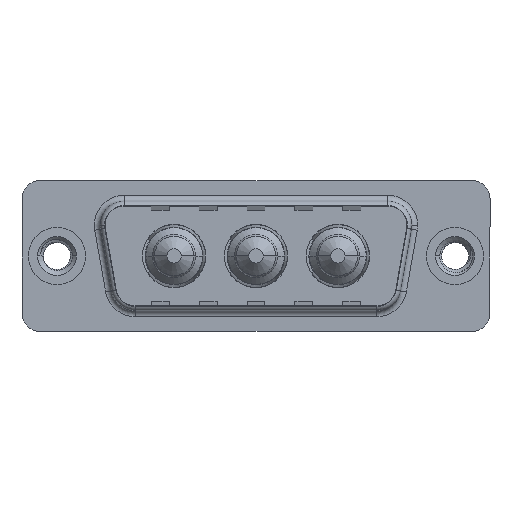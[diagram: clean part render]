
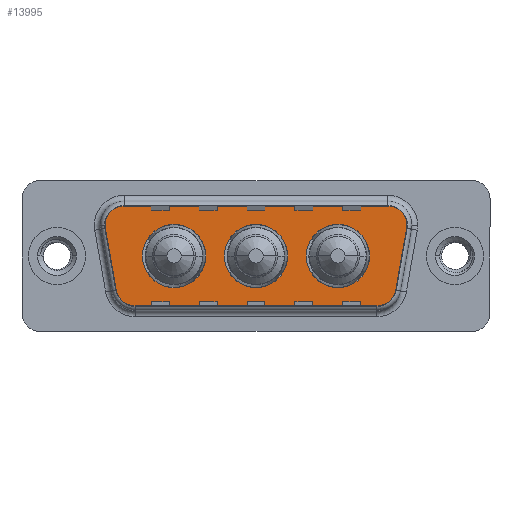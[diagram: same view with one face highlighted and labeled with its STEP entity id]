
A CAD part, top view. The second image highlights one B-rep face of the part: STEP entity #13995.
In plain terms, the highlighted planar face has unit normal (0, 0, 1).
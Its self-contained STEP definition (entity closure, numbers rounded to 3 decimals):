
#9 = CARTESIAN_POINT ( 'NONE',  ( 16.65, 0., 0. ) ) ;
#160 = ORIENTED_EDGE ( 'NONE', *, *, #9346, .F. ) ;
#210 = CARTESIAN_POINT ( 'NONE',  ( 5.411, 4.9, 0. ) ) ;
#265 = DIRECTION ( 'NONE',  ( -1., 0., 0. ) ) ;
#535 = VECTOR ( 'NONE', #265, 1000. ) ;
#558 = CARTESIAN_POINT ( 'NONE',  ( 6.434, -4.9, 0. ) ) ;
#562 = ORIENTED_EDGE ( 'NONE', *, *, #14054, .F. ) ;
#684 = CARTESIAN_POINT ( 'NONE',  ( 26.866, -4.9, 0. ) ) ;
#723 = DIRECTION ( 'NONE',  ( 0., 0., 1. ) ) ;
#787 = CIRCLE ( 'NONE', #1779, 2. ) ;
#826 = DIRECTION ( 'NONE',  ( 0.174, 0.985, 0. ) ) ;
#1057 = AXIS2_PLACEMENT_3D ( 'NONE', #14689, #14650, #14646 ) ;
#1216 = VECTOR ( 'NONE', #826, 1000. ) ;
#1228 = CIRCLE ( 'NONE', #1946, 2. ) ;
#1243 = ORIENTED_EDGE ( 'NONE', *, *, #7879, .F. ) ;
#1320 = CARTESIAN_POINT ( 'NONE',  ( 27.889, 4.9, 0. ) ) ;
#1779 = AXIS2_PLACEMENT_3D ( 'NONE', #15324, #15310, #15288 ) ;
#1879 = DIRECTION ( 'NONE',  ( 1., 0., 0. ) ) ;
#1946 = AXIS2_PLACEMENT_3D ( 'NONE', #11433, #4118, #12653 ) ;
#2027 = CARTESIAN_POINT ( 'NONE',  ( 29.859, 2.553, 0. ) ) ;
#2091 = DIRECTION ( 'NONE',  ( 0., 0., 1. ) ) ;
#2092 = ORIENTED_EDGE ( 'NONE', *, *, #9928, .T. ) ;
#2389 = CARTESIAN_POINT ( 'NONE',  ( 5.411, 2.9, 0. ) ) ;
#2414 = ORIENTED_EDGE ( 'NONE', *, *, #2459, .F. ) ;
#2451 = CIRCLE ( 'NONE', #11569, 2.65 ) ;
#2459 = EDGE_CURVE ( 'NONE', #6737, #3568, #2959, .T. ) ;
#2543 = AXIS2_PLACEMENT_3D ( 'NONE', #2389, #6578, #6451 ) ;
#2721 = CARTESIAN_POINT ( 'NONE',  ( 26.15, 0., 0. ) ) ;
#2831 = DIRECTION ( 'NONE',  ( 0., 0., 1. ) ) ;
#2881 = AXIS2_PLACEMENT_3D ( 'NONE', #9, #5529, #13984 ) ;
#2959 = CIRCLE ( 'NONE', #15672, 2.65 ) ;
#3270 = VERTEX_POINT ( 'NONE', #15400 ) ;
#3435 = LINE ( 'NONE', #210, #535 ) ;
#3568 = VERTEX_POINT ( 'NONE', #5178 ) ;
#3673 = VERTEX_POINT ( 'NONE', #5224 ) ;
#3824 = CIRCLE ( 'NONE', #2881, 2.65 ) ;
#3828 = EDGE_LOOP ( 'NONE', ( #7316, #160 ) ) ;
#4067 = CARTESIAN_POINT ( 'NONE',  ( 3.441, 2.553, 0. ) ) ;
#4118 = DIRECTION ( 'NONE',  ( 0., 0., 1. ) ) ;
#4193 = ORIENTED_EDGE ( 'NONE', *, *, #6285, .T. ) ;
#4564 = FACE_BOUND ( 'NONE', #13454, .T. ) ;
#4695 = ORIENTED_EDGE ( 'NONE', *, *, #15006, .T. ) ;
#4740 = DIRECTION ( 'NONE',  ( 0., 0., 1. ) ) ;
#4900 = LINE ( 'NONE', #2027, #1216 ) ;
#5067 = CARTESIAN_POINT ( 'NONE',  ( 4.464, -3.247, 0. ) ) ;
#5170 = LINE ( 'NONE', #11577, #14444 ) ;
#5178 = CARTESIAN_POINT ( 'NONE',  ( 7.15, 0., 0. ) ) ;
#5224 = CARTESIAN_POINT ( 'NONE',  ( 14., 0., 0. ) ) ;
#5529 = DIRECTION ( 'NONE',  ( 0., 0., 1. ) ) ;
#5687 = CARTESIAN_POINT ( 'NONE',  ( 9.8, 0., 0. ) ) ;
#6285 = EDGE_CURVE ( 'NONE', #8178, #7769, #6385, .T. ) ;
#6385 = CIRCLE ( 'NONE', #2543, 2. ) ;
#6451 = DIRECTION ( 'NONE',  ( 1., 0., 0. ) ) ;
#6578 = DIRECTION ( 'NONE',  ( 0., 0., 1. ) ) ;
#6622 = CARTESIAN_POINT ( 'NONE',  ( 20.85, 0., 0. ) ) ;
#6737 = VERTEX_POINT ( 'NONE', #14676 ) ;
#6766 = CARTESIAN_POINT ( 'NONE',  ( 9.8, 0., 0. ) ) ;
#7316 = ORIENTED_EDGE ( 'NONE', *, *, #11555, .F. ) ;
#7460 = EDGE_CURVE ( 'NONE', #11026, #12460, #11541, .T. ) ;
#7506 = EDGE_LOOP ( 'NONE', ( #2414, #562 ) ) ;
#7604 = CARTESIAN_POINT ( 'NONE',  ( 5.411, 4.9, 0. ) ) ;
#7656 = ORIENTED_EDGE ( 'NONE', *, *, #11028, .T. ) ;
#7769 = VERTEX_POINT ( 'NONE', #4067 ) ;
#7793 = EDGE_CURVE ( 'NONE', #10561, #12694, #787, .T. ) ;
#7811 = FACE_BOUND ( 'NONE', #7506, .T. ) ;
#7879 = EDGE_CURVE ( 'NONE', #3673, #3270, #12298, .T. ) ;
#8046 = DIRECTION ( 'NONE',  ( 1., 0., 0. ) ) ;
#8098 = CARTESIAN_POINT ( 'NONE',  ( 23.5, 0., 0. ) ) ;
#8178 = VERTEX_POINT ( 'NONE', #7604 ) ;
#8218 = FACE_OUTER_BOUND ( 'NONE', #14787, .T. ) ;
#8435 = VERTEX_POINT ( 'NONE', #2721 ) ;
#8458 = ORIENTED_EDGE ( 'NONE', *, *, #14545, .T. ) ;
#8600 = FACE_BOUND ( 'NONE', #3828, .T. ) ;
#8952 = PLANE ( 'NONE',  #14253 ) ;
#9040 = VERTEX_POINT ( 'NONE', #6622 ) ;
#9142 = CIRCLE ( 'NONE', #9356, 2. ) ;
#9193 = VERTEX_POINT ( 'NONE', #1320 ) ;
#9204 = AXIS2_PLACEMENT_3D ( 'NONE', #13824, #13725, #13697 ) ;
#9298 = DIRECTION ( 'NONE',  ( 1., 0., 0. ) ) ;
#9346 = EDGE_CURVE ( 'NONE', #9040, #8435, #11849, .T. ) ;
#9356 = AXIS2_PLACEMENT_3D ( 'NONE', #12038, #4740, #13241 ) ;
#9700 = VERTEX_POINT ( 'NONE', #13318 ) ;
#9919 = VECTOR ( 'NONE', #1879, 1000. ) ;
#9928 = EDGE_CURVE ( 'NONE', #7769, #10561, #5170, .T. ) ;
#9955 = VERTEX_POINT ( 'NONE', #11486 ) ;
#10129 = CARTESIAN_POINT ( 'NONE',  ( 26.866, -2.9, 0. ) ) ;
#10206 = ORIENTED_EDGE ( 'NONE', *, *, #7793, .T. ) ;
#10482 = CARTESIAN_POINT ( 'NONE',  ( 28.836, -3.247, 0. ) ) ;
#10561 = VERTEX_POINT ( 'NONE', #5067 ) ;
#10887 = ORIENTED_EDGE ( 'NONE', *, *, #14657, .T. ) ;
#11026 = VERTEX_POINT ( 'NONE', #684 ) ;
#11028 = EDGE_CURVE ( 'NONE', #12694, #11026, #13148, .T. ) ;
#11049 = EDGE_CURVE ( 'NONE', #9193, #8178, #3435, .T. ) ;
#11053 = ORIENTED_EDGE ( 'NONE', *, *, #11049, .T. ) ;
#11063 = EDGE_CURVE ( 'NONE', #3270, #3673, #3824, .T. ) ;
#11163 = ORIENTED_EDGE ( 'NONE', *, *, #11063, .F. ) ;
#11433 = CARTESIAN_POINT ( 'NONE',  ( 27.889, 2.9, 0. ) ) ;
#11446 = CIRCLE ( 'NONE', #15084, 2.65 ) ;
#11486 = CARTESIAN_POINT ( 'NONE',  ( 29.889, 2.9, 0. ) ) ;
#11539 = DIRECTION ( 'NONE',  ( 0.174, -0.985, 0. ) ) ;
#11541 = CIRCLE ( 'NONE', #13609, 2. ) ;
#11555 = EDGE_CURVE ( 'NONE', #8435, #9040, #2451, .T. ) ;
#11569 = AXIS2_PLACEMENT_3D ( 'NONE', #8098, #723, #9298 ) ;
#11577 = CARTESIAN_POINT ( 'NONE',  ( 3.441, 2.553, 0. ) ) ;
#11587 = DIRECTION ( 'NONE',  ( 1., 0., 0. ) ) ;
#11849 = CIRCLE ( 'NONE', #1057, 2.65 ) ;
#12038 = CARTESIAN_POINT ( 'NONE',  ( 27.889, 2.9, 0. ) ) ;
#12228 = ORIENTED_EDGE ( 'NONE', *, *, #7460, .T. ) ;
#12298 = CIRCLE ( 'NONE', #9204, 2.65 ) ;
#12460 = VERTEX_POINT ( 'NONE', #10482 ) ;
#12653 = DIRECTION ( 'NONE',  ( -1., 0., 0. ) ) ;
#12694 = VERTEX_POINT ( 'NONE', #14528 ) ;
#13148 = LINE ( 'NONE', #558, #9919 ) ;
#13241 = DIRECTION ( 'NONE',  ( -1., 0., 0. ) ) ;
#13318 = CARTESIAN_POINT ( 'NONE',  ( 29.859, 2.553, 0. ) ) ;
#13454 = EDGE_LOOP ( 'NONE', ( #11163, #1243 ) ) ;
#13609 = AXIS2_PLACEMENT_3D ( 'NONE', #14417, #14235, #14141 ) ;
#13697 = DIRECTION ( 'NONE',  ( 1., 0., 0. ) ) ;
#13725 = DIRECTION ( 'NONE',  ( 0., 0., 1. ) ) ;
#13824 = CARTESIAN_POINT ( 'NONE',  ( 16.65, 0., 0. ) ) ;
#13984 = DIRECTION ( 'NONE',  ( 1., 0., 0. ) ) ;
#13995 = ADVANCED_FACE ( 'NONE', ( #4564, #8600, #7811, #8218 ), #8952, .T. ) ;
#14054 = EDGE_CURVE ( 'NONE', #3568, #6737, #11446, .T. ) ;
#14141 = DIRECTION ( 'NONE',  ( 1., 0., 0. ) ) ;
#14235 = DIRECTION ( 'NONE',  ( 0., 0., 1. ) ) ;
#14253 = AXIS2_PLACEMENT_3D ( 'NONE', #10129, #2831, #11587 ) ;
#14417 = CARTESIAN_POINT ( 'NONE',  ( 26.866, -2.9, 0. ) ) ;
#14444 = VECTOR ( 'NONE', #11539, 1000. ) ;
#14528 = CARTESIAN_POINT ( 'NONE',  ( 6.434, -4.9, 0. ) ) ;
#14545 = EDGE_CURVE ( 'NONE', #9700, #9955, #1228, .T. ) ;
#14646 = DIRECTION ( 'NONE',  ( 1., 0., 0. ) ) ;
#14650 = DIRECTION ( 'NONE',  ( 0., 0., 1. ) ) ;
#14657 = EDGE_CURVE ( 'NONE', #9955, #9193, #9142, .T. ) ;
#14676 = CARTESIAN_POINT ( 'NONE',  ( 12.45, 0., 0. ) ) ;
#14689 = CARTESIAN_POINT ( 'NONE',  ( 23.5, 0., 0. ) ) ;
#14787 = EDGE_LOOP ( 'NONE', ( #12228, #4695, #8458, #10887, #11053, #4193, #2092, #10206, #7656 ) ) ;
#15006 = EDGE_CURVE ( 'NONE', #12460, #9700, #4900, .T. ) ;
#15084 = AXIS2_PLACEMENT_3D ( 'NONE', #6766, #15232, #8046 ) ;
#15232 = DIRECTION ( 'NONE',  ( 0., 0., 1. ) ) ;
#15288 = DIRECTION ( 'NONE',  ( -1., 0., 0. ) ) ;
#15310 = DIRECTION ( 'NONE',  ( 0., 0., 1. ) ) ;
#15324 = CARTESIAN_POINT ( 'NONE',  ( 6.434, -2.9, 0. ) ) ;
#15400 = CARTESIAN_POINT ( 'NONE',  ( 19.3, 0., 0. ) ) ;
#15669 = DIRECTION ( 'NONE',  ( 1., 0., 0. ) ) ;
#15672 = AXIS2_PLACEMENT_3D ( 'NONE', #5687, #2091, #15669 ) ;
